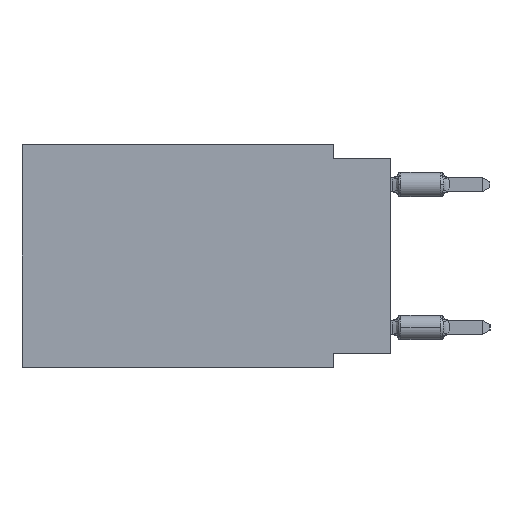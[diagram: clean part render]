
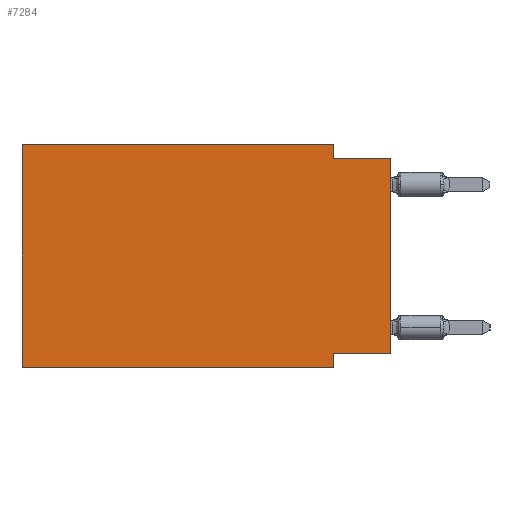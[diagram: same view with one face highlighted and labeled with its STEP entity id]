
A CAD part, left-side view. The second image highlights one B-rep face of the part: STEP entity #7284.
In plain terms, the highlighted planar face has unit normal (-1, 0, 0).
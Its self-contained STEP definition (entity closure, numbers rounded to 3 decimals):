
#26 = LINE ( 'NONE', #14017, #19276 ) ;
#515 = EDGE_CURVE ( 'NONE', #31048, #31743, #29484, .T. ) ;
#1101 = ORIENTED_EDGE ( 'NONE', *, *, #32256, .F. ) ;
#1318 = VERTEX_POINT ( 'NONE', #20806 ) ;
#1375 = ORIENTED_EDGE ( 'NONE', *, *, #23118, .F. ) ;
#1757 = DIRECTION ( 'NONE',  ( 0., 0., -1. ) ) ;
#2000 = VECTOR ( 'NONE', #29658, 1000. ) ;
#2154 = VERTEX_POINT ( 'NONE', #20897 ) ;
#3891 = ORIENTED_EDGE ( 'NONE', *, *, #19821, .T. ) ;
#3942 = CARTESIAN_POINT ( 'NONE',  ( 0., 16.383, -9.906 ) ) ;
#4928 = DIRECTION ( 'NONE',  ( 0., 0., 1. ) ) ;
#7284 = ADVANCED_FACE ( 'NONE', ( #18655 ), #35115, .F. ) ;
#7757 = VECTOR ( 'NONE', #4928, 1000. ) ;
#8788 = DIRECTION ( 'NONE',  ( 0., -1., 0. ) ) ;
#9612 = AXIS2_PLACEMENT_3D ( 'NONE', #18472, #15794, #10796 ) ;
#9988 = CARTESIAN_POINT ( 'NONE',  ( 0., 0., 0. ) ) ;
#10106 = LINE ( 'NONE', #29230, #10627 ) ;
#10369 = ORIENTED_EDGE ( 'NONE', *, *, #22694, .F. ) ;
#10627 = VECTOR ( 'NONE', #34959, 1000. ) ;
#10796 = DIRECTION ( 'NONE',  ( 0., 0., -1. ) ) ;
#10965 = DIRECTION ( 'NONE',  ( 0., 1., 0. ) ) ;
#11488 = VECTOR ( 'NONE', #8788, 1000. ) ;
#11773 = VECTOR ( 'NONE', #26014, 1000. ) ;
#13001 = EDGE_CURVE ( 'NONE', #31048, #24118, #26, .T. ) ;
#14017 = CARTESIAN_POINT ( 'NONE',  ( 0., 0., -9.271 ) ) ;
#14221 = ORIENTED_EDGE ( 'NONE', *, *, #23813, .F. ) ;
#14512 = CARTESIAN_POINT ( 'NONE',  ( 0., 16.383, 0. ) ) ;
#15383 = EDGE_LOOP ( 'NONE', ( #18938, #10369, #1375, #14221, #17035, #3891, #1101, #17541 ) ) ;
#15413 = DIRECTION ( 'NONE',  ( 0., -1., 0. ) ) ;
#15794 = DIRECTION ( 'NONE',  ( 1., 0., 0. ) ) ;
#16132 = LINE ( 'NONE', #24191, #18830 ) ;
#16852 = VERTEX_POINT ( 'NONE', #28251 ) ;
#17035 = ORIENTED_EDGE ( 'NONE', *, *, #32032, .F. ) ;
#17541 = ORIENTED_EDGE ( 'NONE', *, *, #13001, .F. ) ;
#18411 = LINE ( 'NONE', #21279, #35399 ) ;
#18472 = CARTESIAN_POINT ( 'NONE',  ( 0., 16.383, 0. ) ) ;
#18655 = FACE_OUTER_BOUND ( 'NONE', #15383, .T. ) ;
#18830 = VECTOR ( 'NONE', #15413, 1000. ) ;
#18938 = ORIENTED_EDGE ( 'NONE', *, *, #515, .T. ) ;
#19125 = CARTESIAN_POINT ( 'NONE',  ( 0., 2.54, -0.635 ) ) ;
#19276 = VECTOR ( 'NONE', #10965, 1000. ) ;
#19442 = CARTESIAN_POINT ( 'NONE',  ( 0., 2.54, -9.271 ) ) ;
#19821 = EDGE_CURVE ( 'NONE', #26339, #1318, #10106, .T. ) ;
#19947 = CARTESIAN_POINT ( 'NONE',  ( 0., 2.54, -9.906 ) ) ;
#20806 = CARTESIAN_POINT ( 'NONE',  ( 0., 2.54, -9.906 ) ) ;
#20897 = CARTESIAN_POINT ( 'NONE',  ( 0., 16.383, 0. ) ) ;
#21279 = CARTESIAN_POINT ( 'NONE',  ( 0., 2.54, 0. ) ) ;
#21742 = LINE ( 'NONE', #26943, #7757 ) ;
#22148 = VERTEX_POINT ( 'NONE', #19125 ) ;
#22324 = CARTESIAN_POINT ( 'NONE',  ( 0., 0., -9.271 ) ) ;
#22694 = EDGE_CURVE ( 'NONE', #22148, #31743, #16132, .T. ) ;
#23118 = EDGE_CURVE ( 'NONE', #16852, #22148, #18411, .T. ) ;
#23813 = EDGE_CURVE ( 'NONE', #2154, #16852, #25592, .T. ) ;
#24118 = VERTEX_POINT ( 'NONE', #19442 ) ;
#24191 = CARTESIAN_POINT ( 'NONE',  ( 0., 0., -0.635 ) ) ;
#25592 = LINE ( 'NONE', #14512, #11488 ) ;
#26014 = DIRECTION ( 'NONE',  ( 0., 0., -1. ) ) ;
#26339 = VERTEX_POINT ( 'NONE', #3942 ) ;
#26943 = CARTESIAN_POINT ( 'NONE',  ( 0., 16.383, 0. ) ) ;
#28251 = CARTESIAN_POINT ( 'NONE',  ( 0., 2.54, 0. ) ) ;
#29230 = CARTESIAN_POINT ( 'NONE',  ( 0., 16.383, -9.906 ) ) ;
#29484 = LINE ( 'NONE', #9988, #2000 ) ;
#29658 = DIRECTION ( 'NONE',  ( 0., 0., 1. ) ) ;
#31048 = VERTEX_POINT ( 'NONE', #22324 ) ;
#31743 = VERTEX_POINT ( 'NONE', #33063 ) ;
#32032 = EDGE_CURVE ( 'NONE', #26339, #2154, #21742, .T. ) ;
#32256 = EDGE_CURVE ( 'NONE', #24118, #1318, #33884, .T. ) ;
#33063 = CARTESIAN_POINT ( 'NONE',  ( 0., 0., -0.635 ) ) ;
#33884 = LINE ( 'NONE', #19947, #11773 ) ;
#34959 = DIRECTION ( 'NONE',  ( 0., -1., 0. ) ) ;
#35115 = PLANE ( 'NONE',  #9612 ) ;
#35399 = VECTOR ( 'NONE', #1757, 1000. ) ;
